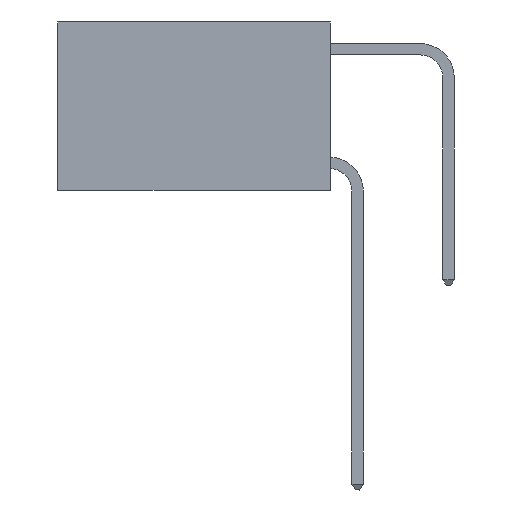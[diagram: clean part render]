
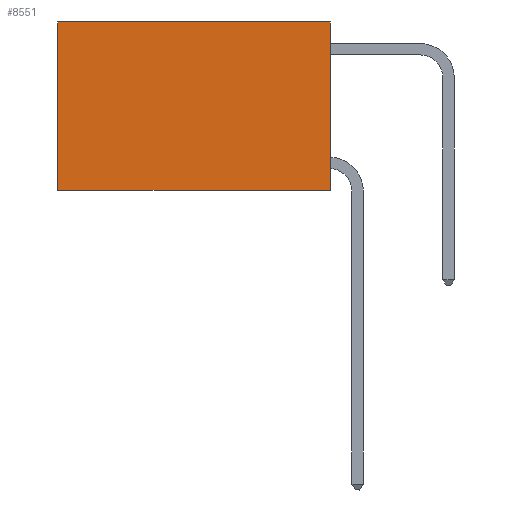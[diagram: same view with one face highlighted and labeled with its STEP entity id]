
A CAD part, left-side view. The second image highlights one B-rep face of the part: STEP entity #8551.
In plain terms, the highlighted planar face has unit normal (-1, 0, 0).
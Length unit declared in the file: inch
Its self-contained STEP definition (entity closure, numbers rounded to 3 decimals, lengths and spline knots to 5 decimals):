
#217 = CARTESIAN_POINT ( 'NONE',  ( 0.2625, 0., -0.37 ) ) ;
#275 = DIRECTION ( 'NONE',  ( 0., 1., 0. ) ) ;
#1345 = DIRECTION ( 'NONE',  ( 0., 1., 0. ) ) ;
#1352 = CARTESIAN_POINT ( 'NONE',  ( 0.2625, 0.6, 0. ) ) ;
#1503 = CARTESIAN_POINT ( 'NONE',  ( 0.2625, 0.6, 0. ) ) ;
#1593 = ORIENTED_EDGE ( 'NONE', *, *, #10670, .F. ) ;
#1686 = VECTOR ( 'NONE', #17477, 39.37008 ) ;
#2249 = VERTEX_POINT ( 'NONE', #1352 ) ;
#3084 = CARTESIAN_POINT ( 'NONE',  ( 0.2625, 0., 0. ) ) ;
#3137 = EDGE_LOOP ( 'NONE', ( #13467, #1593, #6942, #15670 ) ) ;
#3185 = CARTESIAN_POINT ( 'NONE',  ( 0.2625, 0., 0. ) ) ;
#3284 = VERTEX_POINT ( 'NONE', #3084 ) ;
#6942 = ORIENTED_EDGE ( 'NONE', *, *, #7781, .F. ) ;
#7246 = DIRECTION ( 'NONE',  ( 0., 0., -1. ) ) ;
#7467 = VECTOR ( 'NONE', #275, 39.37008 ) ;
#7781 = EDGE_CURVE ( 'NONE', #3284, #13604, #8963, .T. ) ;
#8551 = ADVANCED_FACE ( 'NONE', ( #17269 ), #23102, .F. ) ;
#8963 = LINE ( 'NONE', #11161, #13646 ) ;
#10382 = VERTEX_POINT ( 'NONE', #23520 ) ;
#10670 = EDGE_CURVE ( 'NONE', #13604, #10382, #23966, .T. ) ;
#11161 = CARTESIAN_POINT ( 'NONE',  ( 0.2625, 0., 0. ) ) ;
#11212 = AXIS2_PLACEMENT_3D ( 'NONE', #3185, #19198, #7246 ) ;
#13467 = ORIENTED_EDGE ( 'NONE', *, *, #17117, .T. ) ;
#13604 = VERTEX_POINT ( 'NONE', #217 ) ;
#13646 = VECTOR ( 'NONE', #25030, 39.37008 ) ;
#14050 = VECTOR ( 'NONE', #1345, 39.37008 ) ;
#15340 = CARTESIAN_POINT ( 'NONE',  ( 0.2625, 0., 0. ) ) ;
#15670 = ORIENTED_EDGE ( 'NONE', *, *, #21504, .T. ) ;
#16339 = CARTESIAN_POINT ( 'NONE',  ( 0.2625, 0., -0.37 ) ) ;
#17117 = EDGE_CURVE ( 'NONE', #2249, #10382, #23569, .T. ) ;
#17269 = FACE_OUTER_BOUND ( 'NONE', #3137, .T. ) ;
#17477 = DIRECTION ( 'NONE',  ( 0., 0., -1. ) ) ;
#19198 = DIRECTION ( 'NONE',  ( 1., 0., 0. ) ) ;
#19367 = LINE ( 'NONE', #15340, #14050 ) ;
#21504 = EDGE_CURVE ( 'NONE', #3284, #2249, #19367, .T. ) ;
#23102 = PLANE ( 'NONE',  #11212 ) ;
#23520 = CARTESIAN_POINT ( 'NONE',  ( 0.2625, 0.6, -0.37 ) ) ;
#23569 = LINE ( 'NONE', #1503, #1686 ) ;
#23966 = LINE ( 'NONE', #16339, #7467 ) ;
#25030 = DIRECTION ( 'NONE',  ( 0., 0., -1. ) ) ;
